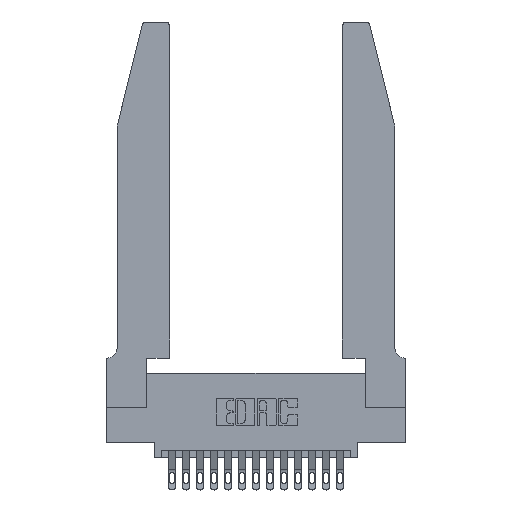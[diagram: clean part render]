
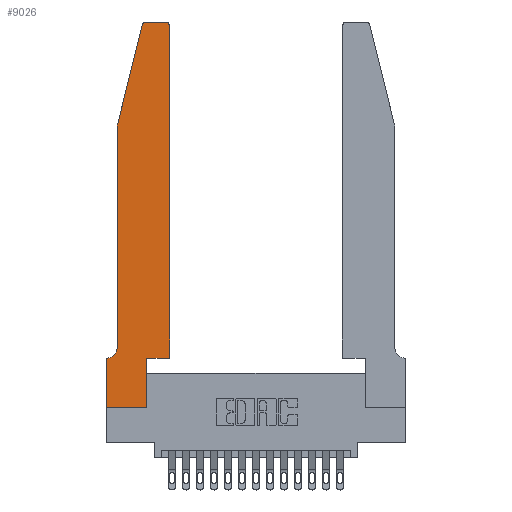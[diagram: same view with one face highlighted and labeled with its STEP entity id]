
A CAD part, top view. The second image highlights one B-rep face of the part: STEP entity #9026.
In plain terms, the highlighted planar face has unit normal (0, 0, 1).
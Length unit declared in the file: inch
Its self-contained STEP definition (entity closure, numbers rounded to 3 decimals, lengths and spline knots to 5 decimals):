
#287 = ORIENTED_EDGE ( 'NONE', *, *, #19293, .T. ) ;
#385 = LINE ( 'NONE', #10281, #8241 ) ;
#882 = DIRECTION ( 'NONE',  ( 0., -1., 0. ) ) ;
#1104 = VERTEX_POINT ( 'NONE', #3993 ) ;
#1132 = AXIS2_PLACEMENT_3D ( 'NONE', #12648, #15364, #10993 ) ;
#1270 = CARTESIAN_POINT ( 'NONE',  ( 0.4505, 0.35, 0.37 ) ) ;
#1381 = LINE ( 'NONE', #11602, #13022 ) ;
#1739 = FACE_OUTER_BOUND ( 'NONE', #2823, .T. ) ;
#1948 = PLANE ( 'NONE',  #9417 ) ;
#2249 = LINE ( 'NONE', #6024, #17094 ) ;
#2284 = CARTESIAN_POINT ( 'NONE',  ( 0.0055, 0.35, 0.37 ) ) ;
#2787 = EDGE_CURVE ( 'NONE', #19271, #5634, #12038, .T. ) ;
#2823 = EDGE_LOOP ( 'NONE', ( #7907, #7977, #8427, #3326, #3859, #11431, #4155, #12402, #15709, #3088, #7820, #287 ) ) ;
#2959 = CARTESIAN_POINT ( 'NONE',  ( 0.25487, 2.72718, 0.37 ) ) ;
#2972 = CARTESIAN_POINT ( 'NONE',  ( 0.0755, 0.42, 0.37 ) ) ;
#3088 = ORIENTED_EDGE ( 'NONE', *, *, #15211, .T. ) ;
#3135 = VERTEX_POINT ( 'NONE', #2972 ) ;
#3326 = ORIENTED_EDGE ( 'NONE', *, *, #14985, .T. ) ;
#3519 = DIRECTION ( 'NONE',  ( 1., 0., 0. ) ) ;
#3727 = VERTEX_POINT ( 'NONE', #13111 ) ;
#3859 = ORIENTED_EDGE ( 'NONE', *, *, #17183, .T. ) ;
#3993 = CARTESIAN_POINT ( 'NONE',  ( 0.0755, 2., 0.37 ) ) ;
#4048 = DIRECTION ( 'NONE',  ( -1., 0., 0. ) ) ;
#4132 = CARTESIAN_POINT ( 'NONE',  ( 0.4505, 0.35, 0.37 ) ) ;
#4155 = ORIENTED_EDGE ( 'NONE', *, *, #15155, .T. ) ;
#4243 = DIRECTION ( 'NONE',  ( 0., 0., 1. ) ) ;
#4441 = CARTESIAN_POINT ( 'NONE',  ( 0.0755, 0.35, 0.37 ) ) ;
#4926 = CARTESIAN_POINT ( 'NONE',  ( 0.0755, 2., 0.37 ) ) ;
#5002 = LINE ( 'NONE', #4132, #12044 ) ;
#5036 = CARTESIAN_POINT ( 'NONE',  ( 0., 0.35, 0.37 ) ) ;
#5634 = VERTEX_POINT ( 'NONE', #2959 ) ;
#5740 = DIRECTION ( 'NONE',  ( 0., 1., 0. ) ) ;
#6024 = CARTESIAN_POINT ( 'NONE',  ( 0.2865, 0.35, 0.37 ) ) ;
#6059 = VERTEX_POINT ( 'NONE', #15688 ) ;
#6067 = LINE ( 'NONE', #8745, #9611 ) ;
#6342 = EDGE_CURVE ( 'NONE', #16410, #3727, #11919, .T. ) ;
#6534 = DIRECTION ( 'NONE',  ( 0., -1., 0. ) ) ;
#6932 = VERTEX_POINT ( 'NONE', #1270 ) ;
#7820 = ORIENTED_EDGE ( 'NONE', *, *, #16517, .T. ) ;
#7907 = ORIENTED_EDGE ( 'NONE', *, *, #12054, .T. ) ;
#7977 = ORIENTED_EDGE ( 'NONE', *, *, #2787, .T. ) ;
#8241 = VECTOR ( 'NONE', #18849, 39.37008 ) ;
#8400 = CIRCLE ( 'NONE', #13601, 0.07 ) ;
#8427 = ORIENTED_EDGE ( 'NONE', *, *, #13750, .T. ) ;
#8573 = CARTESIAN_POINT ( 'NONE',  ( 0.4205, 2.75, 0.37 ) ) ;
#8745 = CARTESIAN_POINT ( 'NONE',  ( 0., 0., 0.37 ) ) ;
#9026 = ADVANCED_FACE ( 'NONE', ( #1739 ), #1948, .T. ) ;
#9189 = CARTESIAN_POINT ( 'NONE',  ( 0.0055, 0.42, 0.37 ) ) ;
#9328 = VECTOR ( 'NONE', #14221, 39.37008 ) ;
#9417 = AXIS2_PLACEMENT_3D ( 'NONE', #5036, #12558, #3519 ) ;
#9611 = VECTOR ( 'NONE', #10218, 39.37008 ) ;
#10155 = CARTESIAN_POINT ( 'NONE',  ( 0.2605, 2.75, 0.37 ) ) ;
#10218 = DIRECTION ( 'NONE',  ( 1., 0., 0. ) ) ;
#10281 = CARTESIAN_POINT ( 'NONE',  ( 0.4505, 0.35, 0.37 ) ) ;
#10529 = VERTEX_POINT ( 'NONE', #18247 ) ;
#10567 = DIRECTION ( 'NONE',  ( 0., 1., 0. ) ) ;
#10651 = DIRECTION ( 'NONE',  ( -1., 0., 0. ) ) ;
#10993 = DIRECTION ( 'NONE',  ( 1., 0., 0. ) ) ;
#11399 = CARTESIAN_POINT ( 'NONE',  ( 0.0755, 2., 0.37 ) ) ;
#11431 = ORIENTED_EDGE ( 'NONE', *, *, #6342, .T. ) ;
#11452 = VECTOR ( 'NONE', #6534, 39.37008 ) ;
#11482 = VECTOR ( 'NONE', #13230, 39.37008 ) ;
#11602 = CARTESIAN_POINT ( 'NONE',  ( 0., 0., 0.37 ) ) ;
#11690 = VERTEX_POINT ( 'NONE', #18542 ) ;
#11919 = LINE ( 'NONE', #4441, #11482 ) ;
#12038 = CIRCLE ( 'NONE', #1132, 0.03 ) ;
#12044 = VECTOR ( 'NONE', #5740, 39.37008 ) ;
#12054 = EDGE_CURVE ( 'NONE', #16434, #19271, #13887, .T. ) ;
#12060 = EDGE_CURVE ( 'NONE', #11690, #10529, #6067, .T. ) ;
#12402 = ORIENTED_EDGE ( 'NONE', *, *, #12060, .T. ) ;
#12558 = DIRECTION ( 'NONE',  ( 0., 0., 1. ) ) ;
#12648 = CARTESIAN_POINT ( 'NONE',  ( 0.284, 2.72, 0.37 ) ) ;
#13022 = VECTOR ( 'NONE', #882, 39.37008 ) ;
#13111 = CARTESIAN_POINT ( 'NONE',  ( 0., 0.35, 0.37 ) ) ;
#13136 = VERTEX_POINT ( 'NONE', #15646 ) ;
#13216 = CARTESIAN_POINT ( 'NONE',  ( 0.4205, 2.72, 0.37 ) ) ;
#13230 = DIRECTION ( 'NONE',  ( -1., 0., 0. ) ) ;
#13601 = AXIS2_PLACEMENT_3D ( 'NONE', #9189, #19223, #10651 ) ;
#13750 = EDGE_CURVE ( 'NONE', #5634, #1104, #16903, .T. ) ;
#13887 = LINE ( 'NONE', #10155, #17201 ) ;
#14221 = DIRECTION ( 'NONE',  ( -0.239, -0.971, 0. ) ) ;
#14534 = CARTESIAN_POINT ( 'NONE',  ( 0.284, 2.75, 0.37 ) ) ;
#14649 = DIRECTION ( 'NONE',  ( 1., 0., 0. ) ) ;
#14985 = EDGE_CURVE ( 'NONE', #1104, #3135, #15676, .T. ) ;
#15155 = EDGE_CURVE ( 'NONE', #3727, #11690, #1381, .T. ) ;
#15211 = EDGE_CURVE ( 'NONE', #13136, #6932, #385, .T. ) ;
#15364 = DIRECTION ( 'NONE',  ( 0., 0., 1. ) ) ;
#15646 = CARTESIAN_POINT ( 'NONE',  ( 0.2865, 0.35, 0.37 ) ) ;
#15676 = LINE ( 'NONE', #4926, #11452 ) ;
#15688 = CARTESIAN_POINT ( 'NONE',  ( 0.4505, 2.72, 0.37 ) ) ;
#15709 = ORIENTED_EDGE ( 'NONE', *, *, #18266, .T. ) ;
#16410 = VERTEX_POINT ( 'NONE', #2284 ) ;
#16434 = VERTEX_POINT ( 'NONE', #8573 ) ;
#16517 = EDGE_CURVE ( 'NONE', #6932, #6059, #5002, .T. ) ;
#16903 = LINE ( 'NONE', #11399, #9328 ) ;
#17094 = VECTOR ( 'NONE', #10567, 39.37008 ) ;
#17178 = AXIS2_PLACEMENT_3D ( 'NONE', #13216, #4243, #14649 ) ;
#17183 = EDGE_CURVE ( 'NONE', #3135, #16410, #8400, .T. ) ;
#17201 = VECTOR ( 'NONE', #4048, 39.37008 ) ;
#17778 = CIRCLE ( 'NONE', #17178, 0.03 ) ;
#18247 = CARTESIAN_POINT ( 'NONE',  ( 0.2865, 0., 0.37 ) ) ;
#18266 = EDGE_CURVE ( 'NONE', #10529, #13136, #2249, .T. ) ;
#18542 = CARTESIAN_POINT ( 'NONE',  ( 0., 0., 0.37 ) ) ;
#18849 = DIRECTION ( 'NONE',  ( 1., 0., 0. ) ) ;
#19223 = DIRECTION ( 'NONE',  ( 0., 0., -1. ) ) ;
#19271 = VERTEX_POINT ( 'NONE', #14534 ) ;
#19293 = EDGE_CURVE ( 'NONE', #6059, #16434, #17778, .T. ) ;
